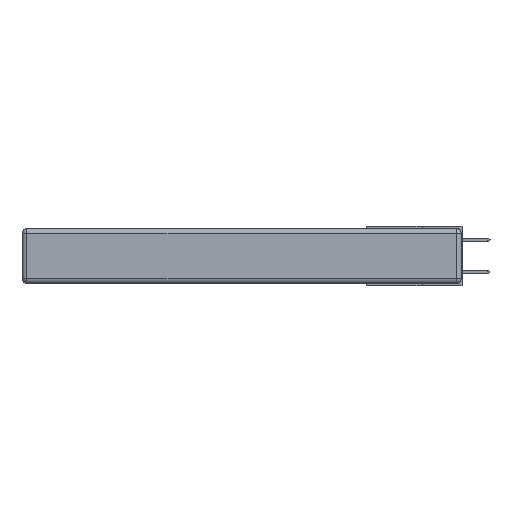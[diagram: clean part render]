
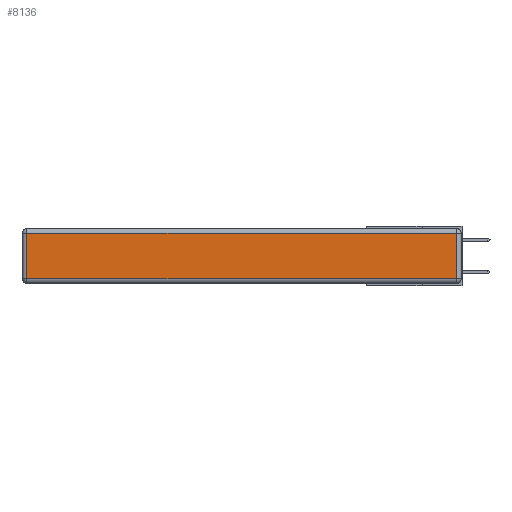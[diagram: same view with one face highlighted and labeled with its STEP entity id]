
A CAD part, left-side view. The second image highlights one B-rep face of the part: STEP entity #8136.
In plain terms, the highlighted planar face has unit normal (-1, 0, 0).
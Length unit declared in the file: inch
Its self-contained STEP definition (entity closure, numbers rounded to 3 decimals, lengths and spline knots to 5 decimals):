
#107 = CARTESIAN_POINT ( 'NONE',  ( 0., 2.72, -0.343 ) ) ;
#998 = CARTESIAN_POINT ( 'NONE',  ( 0., 2.72, -0.03 ) ) ;
#2612 = VERTEX_POINT ( 'NONE', #3424 ) ;
#3424 = CARTESIAN_POINT ( 'NONE',  ( 0., 0.03, -0.313 ) ) ;
#6416 = CARTESIAN_POINT ( 'NONE',  ( 0., 2.72, -0.313 ) ) ;
#6590 = ORIENTED_EDGE ( 'NONE', *, *, #18419, .T. ) ;
#7988 = VECTOR ( 'NONE', #27482, 39.37008 ) ;
#8136 = ADVANCED_FACE ( 'NONE', ( #13059 ), #13585, .T. ) ;
#8953 = DIRECTION ( 'NONE',  ( 0., 1., 0. ) ) ;
#9219 = EDGE_CURVE ( 'NONE', #12736, #2612, #18783, .T. ) ;
#10009 = CARTESIAN_POINT ( 'NONE',  ( 0., 0., -0.313 ) ) ;
#10011 = LINE ( 'NONE', #107, #7988 ) ;
#12639 = EDGE_CURVE ( 'NONE', #2612, #20429, #26709, .T. ) ;
#12736 = VERTEX_POINT ( 'NONE', #6416 ) ;
#13059 = FACE_OUTER_BOUND ( 'NONE', #16871, .T. ) ;
#13585 = PLANE ( 'NONE',  #27767 ) ;
#13599 = CARTESIAN_POINT ( 'NONE',  ( 0., 0.03, -0.03 ) ) ;
#16871 = EDGE_LOOP ( 'NONE', ( #29362, #27953, #32122, #6590 ) ) ;
#17674 = CARTESIAN_POINT ( 'NONE',  ( 0., 0.03, -0.343 ) ) ;
#18405 = DIRECTION ( 'NONE',  ( 0., 0., 1. ) ) ;
#18419 = EDGE_CURVE ( 'NONE', #24230, #12736, #10011, .T. ) ;
#18616 = DIRECTION ( 'NONE',  ( -1., 0., 0. ) ) ;
#18783 = LINE ( 'NONE', #10009, #31202 ) ;
#18878 = LINE ( 'NONE', #28499, #22023 ) ;
#20429 = VERTEX_POINT ( 'NONE', #13599 ) ;
#22023 = VECTOR ( 'NONE', #8953, 39.37008 ) ;
#22287 = DIRECTION ( 'NONE',  ( 0., -1., 0. ) ) ;
#22444 = DIRECTION ( 'NONE',  ( 0., 0., 1. ) ) ;
#24230 = VERTEX_POINT ( 'NONE', #998 ) ;
#25165 = VECTOR ( 'NONE', #22444, 39.37008 ) ;
#26709 = LINE ( 'NONE', #17674, #25165 ) ;
#27482 = DIRECTION ( 'NONE',  ( 0., 0., -1. ) ) ;
#27767 = AXIS2_PLACEMENT_3D ( 'NONE', #30884, #18616, #18405 ) ;
#27953 = ORIENTED_EDGE ( 'NONE', *, *, #12639, .T. ) ;
#28499 = CARTESIAN_POINT ( 'NONE',  ( 0., 2.75, -0.03 ) ) ;
#29228 = EDGE_CURVE ( 'NONE', #20429, #24230, #18878, .T. ) ;
#29362 = ORIENTED_EDGE ( 'NONE', *, *, #9219, .T. ) ;
#30884 = CARTESIAN_POINT ( 'NONE',  ( 0., 0., -0.343 ) ) ;
#31202 = VECTOR ( 'NONE', #22287, 39.37008 ) ;
#32122 = ORIENTED_EDGE ( 'NONE', *, *, #29228, .T. ) ;
